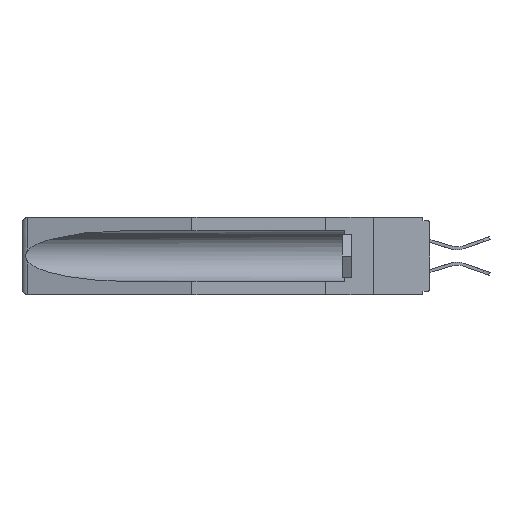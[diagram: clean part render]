
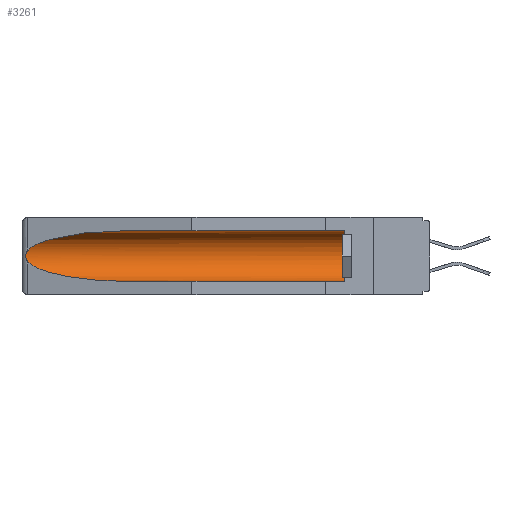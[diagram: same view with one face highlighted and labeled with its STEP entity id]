
A CAD part, left-side view. The second image highlights one B-rep face of the part: STEP entity #3261.
In plain terms, the highlighted cylindrical face has radius 2.857 mm (diameter 5.715 mm), a partial arc.
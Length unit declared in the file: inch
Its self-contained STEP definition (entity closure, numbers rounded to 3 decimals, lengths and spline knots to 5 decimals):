
#808 = CARTESIAN_POINT ( 'NONE',  ( 0.21114, 1.30732, -0.059 ) ) ;
#1205 = AXIS2_PLACEMENT_3D ( 'NONE', #9512, #1397, #18991 ) ;
#1322 = CARTESIAN_POINT ( 'NONE',  ( 0.26537, 1.52718, -0.19328 ) ) ;
#1325 = EDGE_CURVE ( 'NONE', #5039, #2584, #9883, .T. ) ;
#1397 = DIRECTION ( 'NONE',  ( 0., -1., 0. ) ) ;
#1780 = ORIENTED_EDGE ( 'NONE', *, *, #14045, .T. ) ;
#2196 = CARTESIAN_POINT ( 'NONE',  ( 0.155, 1.07973, -0.059 ) ) ;
#2469 = CARTESIAN_POINT ( 'NONE',  ( 0.26537, 1.52718, -0.19328 ) ) ;
#2493 = EDGE_CURVE ( 'NONE', #5039, #13054, #16794, .T. ) ;
#2584 = VERTEX_POINT ( 'NONE', #14545 ) ;
#3261 = ADVANCED_FACE ( 'NONE', ( #19534 ), #10540, .F. ) ;
#3707 = B_SPLINE_CURVE_WITH_KNOTS ( 'NONE', 3,
 ( #18770, #12425, #4559, #20594, #17281, #7788, #15666, #18840, #17141, #1322 ),
 .UNSPECIFIED., .F., .F.,
 ( 4, 2, 2, 2, 4 ),
 ( 0., 0.00029, 0.00058, 0.00087, 0.00117 ),
 .UNSPECIFIED. ) ;
#3719 = ORIENTED_EDGE ( 'NONE', *, *, #2493, .F. ) ;
#3879 = VECTOR ( 'NONE', #18809, 39.37008 ) ;
#4559 = CARTESIAN_POINT ( 'NONE',  ( 0.26654, 1.53092, -0.15636 ) ) ;
#5039 = VERTEX_POINT ( 'NONE', #10943 ) ;
#5475 = VECTOR ( 'NONE', #6546, 39.37008 ) ;
#5595 = DIRECTION ( 'NONE',  ( 0., 1., 0. ) ) ;
#5832 = CARTESIAN_POINT ( 'NONE',  ( 0.25451, 1.48313, -0.24835 ) ) ;
#6546 = DIRECTION ( 'NONE',  ( 0., 1., 0. ) ) ;
#6932 = ORIENTED_EDGE ( 'NONE', *, *, #18534, .T. ) ;
#7686 = CARTESIAN_POINT ( 'NONE',  ( 0.155, -0.30754, -0.284 ) ) ;
#7788 = CARTESIAN_POINT ( 'NONE',  ( 0.2675, 1.53308, -0.17534 ) ) ;
#8328 =( BOUNDED_CURVE ( )  B_SPLINE_CURVE ( 3, ( #16688, #808, #15367, #18586 ),
 .UNSPECIFIED., .F., .F. ) 
 B_SPLINE_CURVE_WITH_KNOTS ( ( 4, 4 ),
 ( 4.71239, 6.08839 ),
 .UNSPECIFIED. ) 
 CURVE ( )  GEOMETRIC_REPRESENTATION_ITEM ( )  RATIONAL_B_SPLINE_CURVE ( ( 1., 0.848, 0.848, 1. ) ) 
 REPRESENTATION_ITEM ( '' )  );
#8424 = EDGE_LOOP ( 'NONE', ( #1780, #13967, #6932, #3719, #9262, #19286 ) ) ;
#8930 = CARTESIAN_POINT ( 'NONE',  ( 0.155, 1.07973, -0.284 ) ) ;
#9262 = ORIENTED_EDGE ( 'NONE', *, *, #1325, .T. ) ;
#9512 = CARTESIAN_POINT ( 'NONE',  ( 0.155, 0.126, -0.1715 ) ) ;
#9883 = CIRCLE ( 'NONE', #1205, 0.1125 ) ;
#10232 =( BOUNDED_CURVE ( )  B_SPLINE_CURVE ( 3, ( #2469, #5832, #19969, #16931 ),
 .UNSPECIFIED., .F., .F. ) 
 B_SPLINE_CURVE_WITH_KNOTS ( ( 4, 4 ),
 ( 0.1948, 1.5708 ),
 .UNSPECIFIED. ) 
 CURVE ( )  GEOMETRIC_REPRESENTATION_ITEM ( )  RATIONAL_B_SPLINE_CURVE ( ( 1., 0.848, 0.848, 1. ) ) 
 REPRESENTATION_ITEM ( '' )  );
#10540 = CYLINDRICAL_SURFACE ( 'NONE', #16305, 0.1125 ) ;
#10943 = CARTESIAN_POINT ( 'NONE',  ( 0.155, 0.126, -0.284 ) ) ;
#11465 = CARTESIAN_POINT ( 'NONE',  ( 0.155, -0.30754, -0.059 ) ) ;
#12133 = EDGE_CURVE ( 'NONE', #2584, #12212, #17377, .T. ) ;
#12212 = VERTEX_POINT ( 'NONE', #2196 ) ;
#12425 = CARTESIAN_POINT ( 'NONE',  ( 0.26597, 1.52961, -0.15275 ) ) ;
#12459 = EDGE_CURVE ( 'NONE', #19826, #17014, #3707, .T. ) ;
#13054 = VERTEX_POINT ( 'NONE', #8930 ) ;
#13967 = ORIENTED_EDGE ( 'NONE', *, *, #12459, .T. ) ;
#14045 = EDGE_CURVE ( 'NONE', #12212, #19826, #8328, .T. ) ;
#14545 = CARTESIAN_POINT ( 'NONE',  ( 0.155, 0.126, -0.059 ) ) ;
#15367 = CARTESIAN_POINT ( 'NONE',  ( 0.25451, 1.48313, -0.09465 ) ) ;
#15666 = CARTESIAN_POINT ( 'NONE',  ( 0.2673, 1.53269, -0.17917 ) ) ;
#16305 = AXIS2_PLACEMENT_3D ( 'NONE', #19879, #5595, #20004 ) ;
#16688 = CARTESIAN_POINT ( 'NONE',  ( 0.155, 1.07973, -0.059 ) ) ;
#16794 = LINE ( 'NONE', #7686, #3879 ) ;
#16931 = CARTESIAN_POINT ( 'NONE',  ( 0.155, 1.07973, -0.284 ) ) ;
#17014 = VERTEX_POINT ( 'NONE', #17343 ) ;
#17141 = CARTESIAN_POINT ( 'NONE',  ( 0.26597, 1.5296, -0.19026 ) ) ;
#17281 = CARTESIAN_POINT ( 'NONE',  ( 0.2675, 1.53308, -0.16763 ) ) ;
#17343 = CARTESIAN_POINT ( 'NONE',  ( 0.26537, 1.52718, -0.19328 ) ) ;
#17377 = LINE ( 'NONE', #11465, #5475 ) ;
#18534 = EDGE_CURVE ( 'NONE', #17014, #13054, #10232, .T. ) ;
#18586 = CARTESIAN_POINT ( 'NONE',  ( 0.26537, 1.52718, -0.14972 ) ) ;
#18613 = CARTESIAN_POINT ( 'NONE',  ( 0.26537, 1.52718, -0.14972 ) ) ;
#18770 = CARTESIAN_POINT ( 'NONE',  ( 0.26537, 1.52718, -0.14972 ) ) ;
#18809 = DIRECTION ( 'NONE',  ( 0., 1., 0. ) ) ;
#18840 = CARTESIAN_POINT ( 'NONE',  ( 0.26655, 1.53094, -0.18657 ) ) ;
#18991 = DIRECTION ( 'NONE',  ( 0., 0., 1. ) ) ;
#19286 = ORIENTED_EDGE ( 'NONE', *, *, #12133, .T. ) ;
#19534 = FACE_OUTER_BOUND ( 'NONE', #8424, .T. ) ;
#19826 = VERTEX_POINT ( 'NONE', #18613 ) ;
#19879 = CARTESIAN_POINT ( 'NONE',  ( 0.155, -0.30754, -0.1715 ) ) ;
#19969 = CARTESIAN_POINT ( 'NONE',  ( 0.21114, 1.30732, -0.284 ) ) ;
#20004 = DIRECTION ( 'NONE',  ( 0., 0., 1. ) ) ;
#20594 = CARTESIAN_POINT ( 'NONE',  ( 0.2673, 1.5327, -0.16383 ) ) ;
